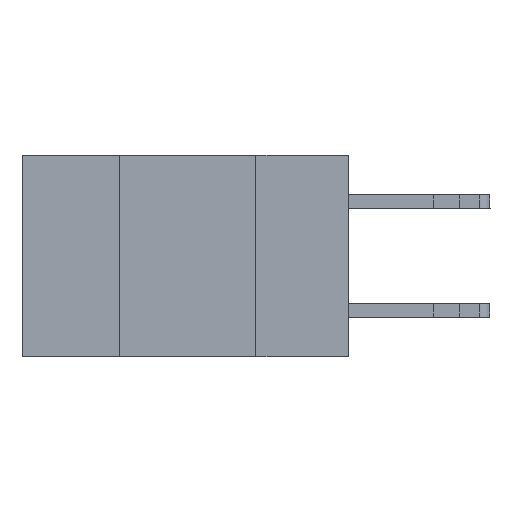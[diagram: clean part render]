
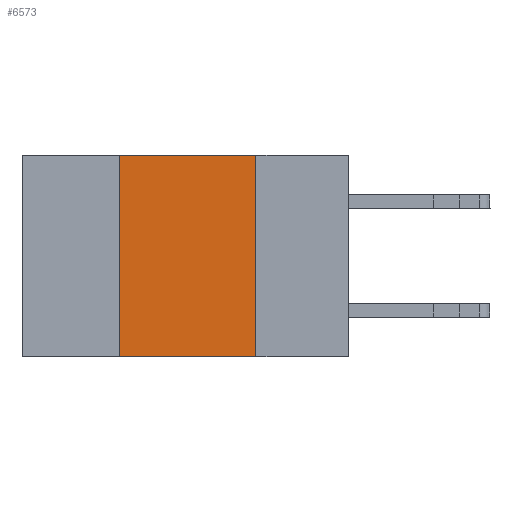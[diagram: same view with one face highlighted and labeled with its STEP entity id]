
A CAD part, left-side view. The second image highlights one B-rep face of the part: STEP entity #6573.
In plain terms, the highlighted planar face has unit normal (-1, 0, 0).
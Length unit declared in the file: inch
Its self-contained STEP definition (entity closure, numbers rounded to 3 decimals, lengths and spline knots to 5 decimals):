
#964 = DIRECTION ( 'NONE',  ( 1., 0., 0. ) ) ;
#1548 = EDGE_CURVE ( 'NONE', #2653, #10829, #4972, .T. ) ;
#1832 = VECTOR ( 'NONE', #7376, 39.37008 ) ;
#2025 = AXIS2_PLACEMENT_3D ( 'NONE', #10853, #964, #5364 ) ;
#2037 = VERTEX_POINT ( 'NONE', #6278 ) ;
#2096 = LINE ( 'NONE', #10918, #1832 ) ;
#2653 = VERTEX_POINT ( 'NONE', #9780 ) ;
#3236 = VERTEX_POINT ( 'NONE', #6209 ) ;
#3955 = LINE ( 'NONE', #8363, #5877 ) ;
#4225 = ORIENTED_EDGE ( 'NONE', *, *, #5128, .F. ) ;
#4972 = LINE ( 'NONE', #11703, #5785 ) ;
#5128 = EDGE_CURVE ( 'NONE', #3236, #2653, #12025, .T. ) ;
#5364 = DIRECTION ( 'NONE',  ( 0., 0., -1. ) ) ;
#5439 = DIRECTION ( 'NONE',  ( 0., 0., 1. ) ) ;
#5785 = VECTOR ( 'NONE', #14006, 39.37008 ) ;
#5877 = VECTOR ( 'NONE', #11695, 39.37008 ) ;
#6209 = CARTESIAN_POINT ( 'NONE',  ( 0., 0.42, -0.37 ) ) ;
#6278 = CARTESIAN_POINT ( 'NONE',  ( 0., 0.17, -0.37 ) ) ;
#6573 = ADVANCED_FACE ( 'NONE', ( #13020 ), #11938, .F. ) ;
#6995 = EDGE_CURVE ( 'NONE', #3236, #2037, #2096, .T. ) ;
#7376 = DIRECTION ( 'NONE',  ( 0., -1., 0. ) ) ;
#7419 = ORIENTED_EDGE ( 'NONE', *, *, #7507, .F. ) ;
#7507 = EDGE_CURVE ( 'NONE', #10829, #2037, #3955, .T. ) ;
#8363 = CARTESIAN_POINT ( 'NONE',  ( 0., 0.17, -0.37 ) ) ;
#9780 = CARTESIAN_POINT ( 'NONE',  ( 0., 0.42, 0. ) ) ;
#9840 = CARTESIAN_POINT ( 'NONE',  ( 0., 0.42, -0.37 ) ) ;
#9978 = CARTESIAN_POINT ( 'NONE',  ( 0., 0.17, 0. ) ) ;
#10119 = ORIENTED_EDGE ( 'NONE', *, *, #1548, .F. ) ;
#10829 = VERTEX_POINT ( 'NONE', #9978 ) ;
#10853 = CARTESIAN_POINT ( 'NONE',  ( 0., 0.6, 0. ) ) ;
#10918 = CARTESIAN_POINT ( 'NONE',  ( 0., 0.6, -0.37 ) ) ;
#11695 = DIRECTION ( 'NONE',  ( 0., 0., -1. ) ) ;
#11703 = CARTESIAN_POINT ( 'NONE',  ( 0., 0.6, 0. ) ) ;
#11938 = PLANE ( 'NONE',  #2025 ) ;
#12025 = LINE ( 'NONE', #9840, #12714 ) ;
#12714 = VECTOR ( 'NONE', #5439, 39.37008 ) ;
#12983 = ORIENTED_EDGE ( 'NONE', *, *, #6995, .T. ) ;
#13020 = FACE_OUTER_BOUND ( 'NONE', #13900, .T. ) ;
#13900 = EDGE_LOOP ( 'NONE', ( #7419, #10119, #4225, #12983 ) ) ;
#14006 = DIRECTION ( 'NONE',  ( 0., -1., 0. ) ) ;
